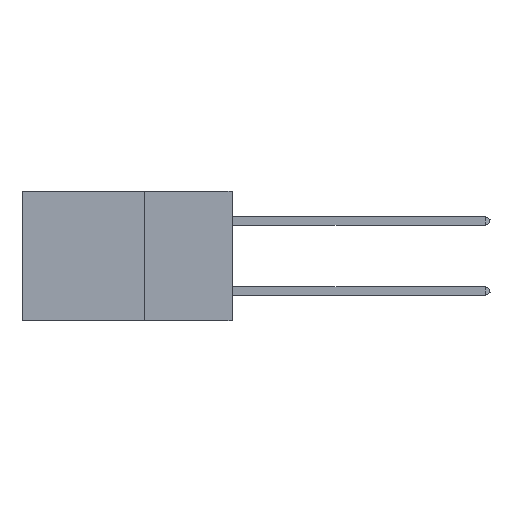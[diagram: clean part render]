
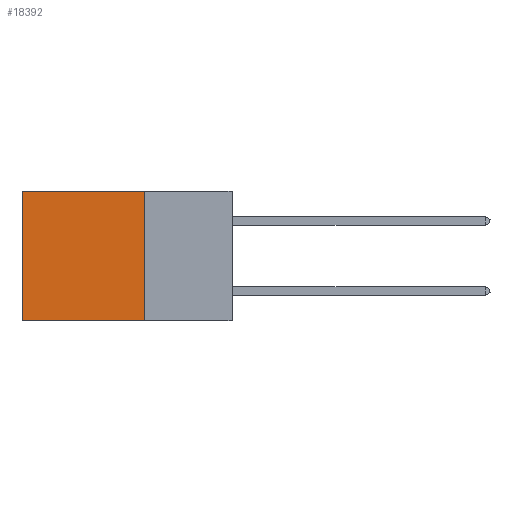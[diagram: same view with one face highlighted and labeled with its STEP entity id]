
A CAD part, left-side view. The second image highlights one B-rep face of the part: STEP entity #18392.
In plain terms, the highlighted planar face has unit normal (-1, 0, 0).
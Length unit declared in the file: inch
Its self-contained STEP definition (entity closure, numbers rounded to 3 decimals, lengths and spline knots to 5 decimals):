
#3372 = CARTESIAN_POINT ( 'NONE',  ( 0.2875, 0.25, 0. ) ) ;
#3813 = VERTEX_POINT ( 'NONE', #31493 ) ;
#4277 = DIRECTION ( 'NONE',  ( 0., 0., -1. ) ) ;
#4432 = CARTESIAN_POINT ( 'NONE',  ( 0.2875, 0.25, 0. ) ) ;
#4562 = EDGE_LOOP ( 'NONE', ( #23936, #9407, #7918, #30136 ) ) ;
#6030 = DIRECTION ( 'NONE',  ( 1., 0., 0. ) ) ;
#6142 = VECTOR ( 'NONE', #7346, 39.37008 ) ;
#7346 = DIRECTION ( 'NONE',  ( 0., 1., 0. ) ) ;
#7412 = DIRECTION ( 'NONE',  ( 0., 1., 0. ) ) ;
#7918 = ORIENTED_EDGE ( 'NONE', *, *, #29274, .F. ) ;
#7980 = VERTEX_POINT ( 'NONE', #31489 ) ;
#9000 = LINE ( 'NONE', #4432, #9792 ) ;
#9407 = ORIENTED_EDGE ( 'NONE', *, *, #12378, .F. ) ;
#9528 = LINE ( 'NONE', #22249, #16295 ) ;
#9792 = VECTOR ( 'NONE', #22394, 39.37008 ) ;
#10512 = AXIS2_PLACEMENT_3D ( 'NONE', #3372, #6030, #26203 ) ;
#12378 = EDGE_CURVE ( 'NONE', #7980, #3813, #24051, .T. ) ;
#13440 = EDGE_CURVE ( 'NONE', #23284, #15852, #31480, .T. ) ;
#13542 = FACE_OUTER_BOUND ( 'NONE', #4562, .T. ) ;
#15852 = VERTEX_POINT ( 'NONE', #25177 ) ;
#16295 = VECTOR ( 'NONE', #4277, 39.37008 ) ;
#18392 = ADVANCED_FACE ( 'NONE', ( #13542 ), #31158, .F. ) ;
#22062 = VECTOR ( 'NONE', #7412, 39.37008 ) ;
#22249 = CARTESIAN_POINT ( 'NONE',  ( 0.2875, 0.6, 0. ) ) ;
#22394 = DIRECTION ( 'NONE',  ( 0., 0., -1. ) ) ;
#22555 = CARTESIAN_POINT ( 'NONE',  ( 0.2875, 0.25, 0. ) ) ;
#23284 = VERTEX_POINT ( 'NONE', #25653 ) ;
#23936 = ORIENTED_EDGE ( 'NONE', *, *, #27439, .T. ) ;
#24051 = LINE ( 'NONE', #28000, #22062 ) ;
#25177 = CARTESIAN_POINT ( 'NONE',  ( 0.2875, 0.6, 0. ) ) ;
#25653 = CARTESIAN_POINT ( 'NONE',  ( 0.2875, 0.25, 0. ) ) ;
#26203 = DIRECTION ( 'NONE',  ( 0., 0., -1. ) ) ;
#27439 = EDGE_CURVE ( 'NONE', #15852, #3813, #9528, .T. ) ;
#28000 = CARTESIAN_POINT ( 'NONE',  ( 0.2875, 0.25, -0.37 ) ) ;
#29274 = EDGE_CURVE ( 'NONE', #23284, #7980, #9000, .T. ) ;
#30136 = ORIENTED_EDGE ( 'NONE', *, *, #13440, .T. ) ;
#31158 = PLANE ( 'NONE',  #10512 ) ;
#31480 = LINE ( 'NONE', #22555, #6142 ) ;
#31489 = CARTESIAN_POINT ( 'NONE',  ( 0.2875, 0.25, -0.37 ) ) ;
#31493 = CARTESIAN_POINT ( 'NONE',  ( 0.2875, 0.6, -0.37 ) ) ;
